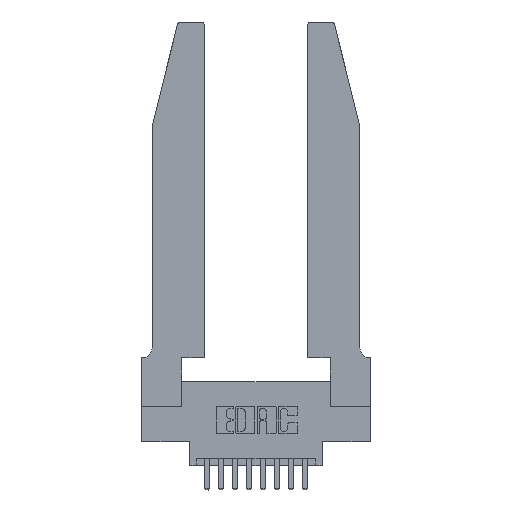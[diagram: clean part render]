
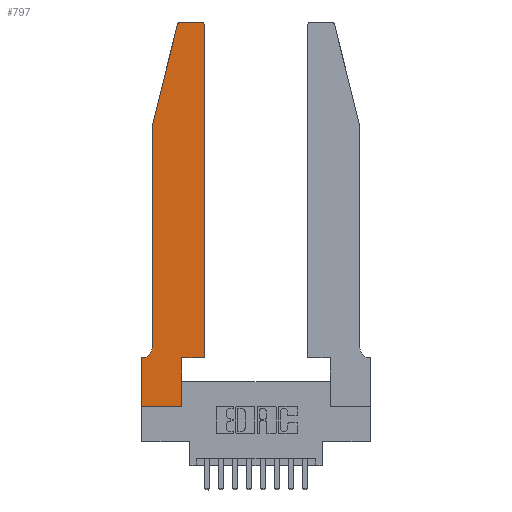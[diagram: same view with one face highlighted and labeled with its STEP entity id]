
A CAD part, top view. The second image highlights one B-rep face of the part: STEP entity #797.
In plain terms, the highlighted planar face has unit normal (0, 0, 1).
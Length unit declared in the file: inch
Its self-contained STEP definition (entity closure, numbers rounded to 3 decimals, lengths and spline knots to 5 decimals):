
#4 = VERTEX_POINT ( 'NONE', #8576 ) ;
#43 = VERTEX_POINT ( 'NONE', #12552 ) ;
#263 = CARTESIAN_POINT ( 'NONE',  ( 0.0055, 0.42, 0.37 ) ) ;
#369 = ORIENTED_EDGE ( 'NONE', *, *, #5400, .T. ) ;
#405 = EDGE_LOOP ( 'NONE', ( #14351, #13732, #1031, #11635, #14929, #14474, #7910, #15192, #369, #9854, #8136, #802 ) ) ;
#600 = EDGE_CURVE ( 'NONE', #3327, #12698, #8341, .T. ) ;
#663 = VECTOR ( 'NONE', #4906, 39.37008 ) ;
#797 = ADVANCED_FACE ( 'NONE', ( #15287 ), #6651, .T. ) ;
#802 = ORIENTED_EDGE ( 'NONE', *, *, #15858, .T. ) ;
#822 = CARTESIAN_POINT ( 'NONE',  ( 0.4505, 2.72, 0.37 ) ) ;
#829 = CARTESIAN_POINT ( 'NONE',  ( 0.2865, 0.35, 0.37 ) ) ;
#1031 = ORIENTED_EDGE ( 'NONE', *, *, #9189, .T. ) ;
#1102 = DIRECTION ( 'NONE',  ( 1., 0., 0. ) ) ;
#1202 = DIRECTION ( 'NONE',  ( -0.239, -0.971, 0. ) ) ;
#1425 = DIRECTION ( 'NONE',  ( 1., 0., 0. ) ) ;
#1518 = DIRECTION ( 'NONE',  ( -1., 0., 0. ) ) ;
#1639 = EDGE_CURVE ( 'NONE', #4775, #6296, #8524, .T. ) ;
#1666 = VECTOR ( 'NONE', #4364, 39.37008 ) ;
#2758 = CARTESIAN_POINT ( 'NONE',  ( 0.0755, 2., 0.37 ) ) ;
#3102 = DIRECTION ( 'NONE',  ( -1., 0., 0. ) ) ;
#3172 = EDGE_CURVE ( 'NONE', #43, #13775, #6553, .T. ) ;
#3312 = VECTOR ( 'NONE', #6288, 39.37008 ) ;
#3327 = VERTEX_POINT ( 'NONE', #6758 ) ;
#3524 = VERTEX_POINT ( 'NONE', #4956 ) ;
#3703 = EDGE_CURVE ( 'NONE', #4, #4775, #5787, .T. ) ;
#3854 = VECTOR ( 'NONE', #1102, 39.37008 ) ;
#3901 = VERTEX_POINT ( 'NONE', #9965 ) ;
#4259 = VERTEX_POINT ( 'NONE', #829 ) ;
#4260 = CARTESIAN_POINT ( 'NONE',  ( 0., 0., 0.37 ) ) ;
#4266 = LINE ( 'NONE', #7395, #663 ) ;
#4364 = DIRECTION ( 'NONE',  ( 0., -1., 0. ) ) ;
#4638 = CARTESIAN_POINT ( 'NONE',  ( 0.284, 2.72, 0.37 ) ) ;
#4698 = DIRECTION ( 'NONE',  ( -1., 0., 0. ) ) ;
#4774 = LINE ( 'NONE', #6488, #7660 ) ;
#4775 = VERTEX_POINT ( 'NONE', #13851 ) ;
#4906 = DIRECTION ( 'NONE',  ( 0., -1., 0. ) ) ;
#4956 = CARTESIAN_POINT ( 'NONE',  ( 0.2865, 0., 0.37 ) ) ;
#5000 = DIRECTION ( 'NONE',  ( 0., 0., 1. ) ) ;
#5400 = EDGE_CURVE ( 'NONE', #3524, #4259, #4774, .T. ) ;
#5787 = LINE ( 'NONE', #6754, #9389 ) ;
#5897 = DIRECTION ( 'NONE',  ( 1., 0., 0. ) ) ;
#6086 = CIRCLE ( 'NONE', #15003, 0.03 ) ;
#6223 = VERTEX_POINT ( 'NONE', #14880 ) ;
#6278 = CARTESIAN_POINT ( 'NONE',  ( 0.4505, 0.35, 0.37 ) ) ;
#6288 = DIRECTION ( 'NONE',  ( 0., 1., 0. ) ) ;
#6296 = VERTEX_POINT ( 'NONE', #10065 ) ;
#6488 = CARTESIAN_POINT ( 'NONE',  ( 0.2865, 0.35, 0.37 ) ) ;
#6553 = LINE ( 'NONE', #6278, #3312 ) ;
#6651 = PLANE ( 'NONE',  #13670 ) ;
#6695 = AXIS2_PLACEMENT_3D ( 'NONE', #4638, #13225, #5897 ) ;
#6754 = CARTESIAN_POINT ( 'NONE',  ( 0.0755, 0.35, 0.37 ) ) ;
#6758 = CARTESIAN_POINT ( 'NONE',  ( 0.4205, 2.75, 0.37 ) ) ;
#7395 = CARTESIAN_POINT ( 'NONE',  ( 0.0755, 2., 0.37 ) ) ;
#7660 = VECTOR ( 'NONE', #8989, 39.37008 ) ;
#7877 = LINE ( 'NONE', #8408, #3854 ) ;
#7910 = ORIENTED_EDGE ( 'NONE', *, *, #1639, .T. ) ;
#7915 = LINE ( 'NONE', #10975, #11170 ) ;
#8136 = ORIENTED_EDGE ( 'NONE', *, *, #3172, .T. ) ;
#8341 = LINE ( 'NONE', #9953, #11215 ) ;
#8397 = VERTEX_POINT ( 'NONE', #2758 ) ;
#8408 = CARTESIAN_POINT ( 'NONE',  ( 0.4505, 0.35, 0.37 ) ) ;
#8524 = LINE ( 'NONE', #4260, #1666 ) ;
#8576 = CARTESIAN_POINT ( 'NONE',  ( 0.0055, 0.35, 0.37 ) ) ;
#8772 = LINE ( 'NONE', #13610, #15326 ) ;
#8800 = DIRECTION ( 'NONE',  ( 0., 0., -1. ) ) ;
#8989 = DIRECTION ( 'NONE',  ( 0., 1., 0. ) ) ;
#9051 = CIRCLE ( 'NONE', #6695, 0.03 ) ;
#9075 = EDGE_CURVE ( 'NONE', #12698, #6223, #9051, .T. ) ;
#9189 = EDGE_CURVE ( 'NONE', #6223, #8397, #7915, .T. ) ;
#9259 = EDGE_CURVE ( 'NONE', #8397, #3901, #4266, .T. ) ;
#9268 = CARTESIAN_POINT ( 'NONE',  ( 0.284, 2.75, 0.37 ) ) ;
#9389 = VECTOR ( 'NONE', #3102, 39.37008 ) ;
#9426 = CIRCLE ( 'NONE', #13138, 0.07 ) ;
#9854 = ORIENTED_EDGE ( 'NONE', *, *, #10716, .T. ) ;
#9953 = CARTESIAN_POINT ( 'NONE',  ( 0.2605, 2.75, 0.37 ) ) ;
#9965 = CARTESIAN_POINT ( 'NONE',  ( 0.0755, 0.42, 0.37 ) ) ;
#10065 = CARTESIAN_POINT ( 'NONE',  ( 0., 0., 0.37 ) ) ;
#10716 = EDGE_CURVE ( 'NONE', #4259, #43, #7877, .T. ) ;
#10975 = CARTESIAN_POINT ( 'NONE',  ( 0.0755, 2., 0.37 ) ) ;
#11170 = VECTOR ( 'NONE', #1202, 39.37008 ) ;
#11215 = VECTOR ( 'NONE', #4698, 39.37008 ) ;
#11635 = ORIENTED_EDGE ( 'NONE', *, *, #9259, .T. ) ;
#12189 = EDGE_CURVE ( 'NONE', #6296, #3524, #8772, .T. ) ;
#12348 = CARTESIAN_POINT ( 'NONE',  ( 0.4205, 2.72, 0.37 ) ) ;
#12552 = CARTESIAN_POINT ( 'NONE',  ( 0.4505, 0.35, 0.37 ) ) ;
#12698 = VERTEX_POINT ( 'NONE', #9268 ) ;
#13138 = AXIS2_PLACEMENT_3D ( 'NONE', #263, #8800, #1518 ) ;
#13225 = DIRECTION ( 'NONE',  ( 0., 0., 1. ) ) ;
#13594 = DIRECTION ( 'NONE',  ( 1., 0., 0. ) ) ;
#13610 = CARTESIAN_POINT ( 'NONE',  ( 0., 0., 0.37 ) ) ;
#13670 = AXIS2_PLACEMENT_3D ( 'NONE', #14938, #15104, #15747 ) ;
#13732 = ORIENTED_EDGE ( 'NONE', *, *, #9075, .T. ) ;
#13775 = VERTEX_POINT ( 'NONE', #822 ) ;
#13851 = CARTESIAN_POINT ( 'NONE',  ( 0., 0.35, 0.37 ) ) ;
#14351 = ORIENTED_EDGE ( 'NONE', *, *, #600, .T. ) ;
#14474 = ORIENTED_EDGE ( 'NONE', *, *, #3703, .T. ) ;
#14880 = CARTESIAN_POINT ( 'NONE',  ( 0.25487, 2.72718, 0.37 ) ) ;
#14929 = ORIENTED_EDGE ( 'NONE', *, *, #15126, .T. ) ;
#14938 = CARTESIAN_POINT ( 'NONE',  ( 0., 0.35, 0.37 ) ) ;
#15003 = AXIS2_PLACEMENT_3D ( 'NONE', #12348, #5000, #13594 ) ;
#15104 = DIRECTION ( 'NONE',  ( 0., 0., 1. ) ) ;
#15126 = EDGE_CURVE ( 'NONE', #3901, #4, #9426, .T. ) ;
#15192 = ORIENTED_EDGE ( 'NONE', *, *, #12189, .T. ) ;
#15287 = FACE_OUTER_BOUND ( 'NONE', #405, .T. ) ;
#15326 = VECTOR ( 'NONE', #1425, 39.37008 ) ;
#15747 = DIRECTION ( 'NONE',  ( 1., 0., 0. ) ) ;
#15858 = EDGE_CURVE ( 'NONE', #13775, #3327, #6086, .T. ) ;
